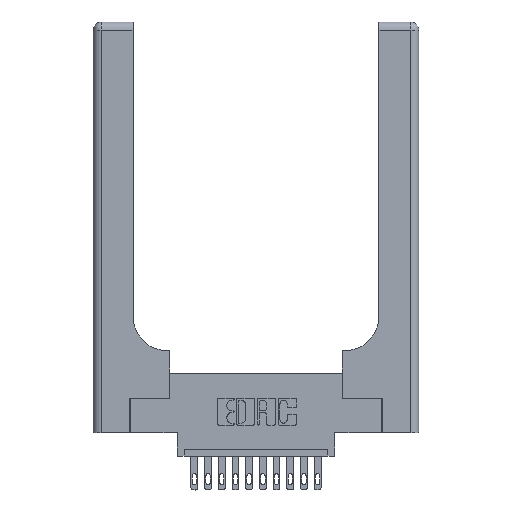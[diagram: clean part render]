
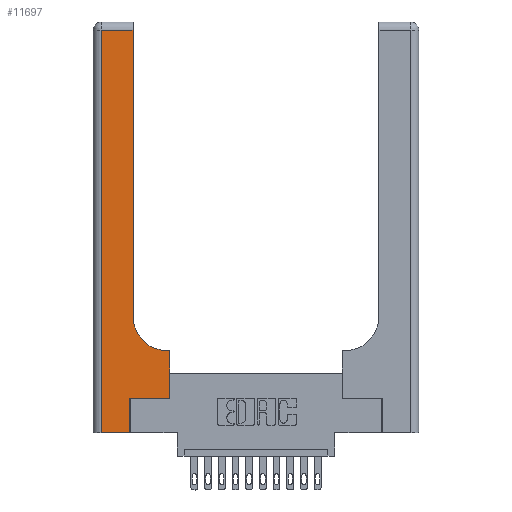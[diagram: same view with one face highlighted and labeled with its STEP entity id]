
A CAD part, top view. The second image highlights one B-rep face of the part: STEP entity #11697.
In plain terms, the highlighted planar face has unit normal (0, 0, 1).
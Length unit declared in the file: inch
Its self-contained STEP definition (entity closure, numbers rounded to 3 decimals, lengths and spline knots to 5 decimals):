
#223 = VECTOR ( 'NONE', #569, 39.37008 ) ;
#533 = ORIENTED_EDGE ( 'NONE', *, *, #6207, .T. ) ;
#569 = DIRECTION ( 'NONE',  ( 0., -1., 0. ) ) ;
#892 = DIRECTION ( 'NONE',  ( 0., 0., -1. ) ) ;
#1038 = CARTESIAN_POINT ( 'NONE',  ( 0.06, 0., 0.37 ) ) ;
#1102 = ORIENTED_EDGE ( 'NONE', *, *, #2010, .T. ) ;
#1997 = DIRECTION ( 'NONE',  ( 0., 1., 0. ) ) ;
#2010 = EDGE_CURVE ( 'NONE', #13955, #14067, #10410, .T. ) ;
#2180 = VECTOR ( 'NONE', #3396, 39.37008 ) ;
#2236 = PLANE ( 'NONE',  #5914 ) ;
#2471 = VERTEX_POINT ( 'NONE', #4602 ) ;
#2488 = DIRECTION ( 'NONE',  ( 0., 1., 0. ) ) ;
#2733 = EDGE_CURVE ( 'NONE', #6774, #13540, #5855, .T. ) ;
#2799 = CARTESIAN_POINT ( 'NONE',  ( 0., 0., 0.37 ) ) ;
#3168 = VERTEX_POINT ( 'NONE', #16794 ) ;
#3284 = VECTOR ( 'NONE', #7440, 39.37008 ) ;
#3396 = DIRECTION ( 'NONE',  ( 0., 1., 0. ) ) ;
#3535 = CARTESIAN_POINT ( 'NONE',  ( 0.5585, 0.25, 0.37 ) ) ;
#3640 = CARTESIAN_POINT ( 'NONE',  ( 0.269, 0., 0.37 ) ) ;
#3785 = CARTESIAN_POINT ( 'NONE',  ( 0.269, 0.25, 0.37 ) ) ;
#3936 = CARTESIAN_POINT ( 'NONE',  ( 0.2915, 2.94, 0.37 ) ) ;
#4176 = DIRECTION ( 'NONE',  ( 1., 0., 0. ) ) ;
#4204 = CARTESIAN_POINT ( 'NONE',  ( 0.2915, 3., 0.37 ) ) ;
#4445 = VERTEX_POINT ( 'NONE', #12158 ) ;
#4602 = CARTESIAN_POINT ( 'NONE',  ( 0.06, 2.94, 0.37 ) ) ;
#4858 = EDGE_CURVE ( 'NONE', #14067, #4445, #7642, .T. ) ;
#5095 = ORIENTED_EDGE ( 'NONE', *, *, #15045, .T. ) ;
#5145 = VECTOR ( 'NONE', #1997, 39.37008 ) ;
#5373 = LINE ( 'NONE', #9634, #223 ) ;
#5727 = EDGE_CURVE ( 'NONE', #13540, #2471, #14902, .T. ) ;
#5855 = LINE ( 'NONE', #4204, #2180 ) ;
#5914 = AXIS2_PLACEMENT_3D ( 'NONE', #8758, #892, #11428 ) ;
#5970 = EDGE_CURVE ( 'NONE', #2471, #6096, #5373, .T. ) ;
#6096 = VERTEX_POINT ( 'NONE', #1038 ) ;
#6207 = EDGE_CURVE ( 'NONE', #11493, #6774, #14070, .T. ) ;
#6405 = VECTOR ( 'NONE', #14387, 39.37008 ) ;
#6507 = VECTOR ( 'NONE', #2488, 39.37008 ) ;
#6774 = VERTEX_POINT ( 'NONE', #12709 ) ;
#7440 = DIRECTION ( 'NONE',  ( -1., 0., 0. ) ) ;
#7642 = LINE ( 'NONE', #13525, #12418 ) ;
#8073 = DIRECTION ( 'NONE',  ( 0., 0., -1. ) ) ;
#8128 = CARTESIAN_POINT ( 'NONE',  ( 0.5415, 0.6, 0.37 ) ) ;
#8676 = CARTESIAN_POINT ( 'NONE',  ( 0.269, 0., 0.37 ) ) ;
#8758 = CARTESIAN_POINT ( 'NONE',  ( 0., 3., 0.37 ) ) ;
#8801 = EDGE_CURVE ( 'NONE', #6096, #13955, #10360, .T. ) ;
#9507 = ORIENTED_EDGE ( 'NONE', *, *, #5970, .T. ) ;
#9634 = CARTESIAN_POINT ( 'NONE',  ( 0.06, 3., 0.37 ) ) ;
#10360 = LINE ( 'NONE', #2799, #11828 ) ;
#10410 = LINE ( 'NONE', #3640, #6507 ) ;
#10461 = CARTESIAN_POINT ( 'NONE',  ( 0., 2.94, 0.37 ) ) ;
#10688 = FACE_OUTER_BOUND ( 'NONE', #14396, .T. ) ;
#10918 = DIRECTION ( 'NONE',  ( 1., 0., 0. ) ) ;
#11428 = DIRECTION ( 'NONE',  ( -1., 0., 0. ) ) ;
#11493 = VERTEX_POINT ( 'NONE', #8128 ) ;
#11602 = CARTESIAN_POINT ( 'NONE',  ( 0.2915, 0.6, 0.37 ) ) ;
#11683 = EDGE_CURVE ( 'NONE', #3168, #11493, #13830, .T. ) ;
#11697 = ADVANCED_FACE ( 'NONE', ( #10688 ), #2236, .F. ) ;
#11828 = VECTOR ( 'NONE', #10918, 39.37008 ) ;
#12158 = CARTESIAN_POINT ( 'NONE',  ( 0.5585, 0.25, 0.37 ) ) ;
#12418 = VECTOR ( 'NONE', #4176, 39.37008 ) ;
#12419 = ORIENTED_EDGE ( 'NONE', *, *, #4858, .T. ) ;
#12546 = ORIENTED_EDGE ( 'NONE', *, *, #8801, .T. ) ;
#12709 = CARTESIAN_POINT ( 'NONE',  ( 0.2915, 0.85, 0.37 ) ) ;
#13032 = AXIS2_PLACEMENT_3D ( 'NONE', #13322, #8073, #13379 ) ;
#13322 = CARTESIAN_POINT ( 'NONE',  ( 0.5415, 0.85, 0.37 ) ) ;
#13379 = DIRECTION ( 'NONE',  ( 1., 0., 0. ) ) ;
#13411 = ORIENTED_EDGE ( 'NONE', *, *, #2733, .T. ) ;
#13525 = CARTESIAN_POINT ( 'NONE',  ( 0.269, 0.25, 0.37 ) ) ;
#13540 = VERTEX_POINT ( 'NONE', #3936 ) ;
#13643 = LINE ( 'NONE', #3535, #5145 ) ;
#13830 = LINE ( 'NONE', #11602, #3284 ) ;
#13955 = VERTEX_POINT ( 'NONE', #8676 ) ;
#14067 = VERTEX_POINT ( 'NONE', #3785 ) ;
#14070 = CIRCLE ( 'NONE', #13032, 0.25 ) ;
#14207 = ORIENTED_EDGE ( 'NONE', *, *, #5727, .T. ) ;
#14387 = DIRECTION ( 'NONE',  ( -1., 0., 0. ) ) ;
#14393 = ORIENTED_EDGE ( 'NONE', *, *, #11683, .T. ) ;
#14396 = EDGE_LOOP ( 'NONE', ( #13411, #14207, #9507, #12546, #1102, #12419, #5095, #14393, #533 ) ) ;
#14902 = LINE ( 'NONE', #10461, #6405 ) ;
#15045 = EDGE_CURVE ( 'NONE', #4445, #3168, #13643, .T. ) ;
#16794 = CARTESIAN_POINT ( 'NONE',  ( 0.5585, 0.6, 0.37 ) ) ;
